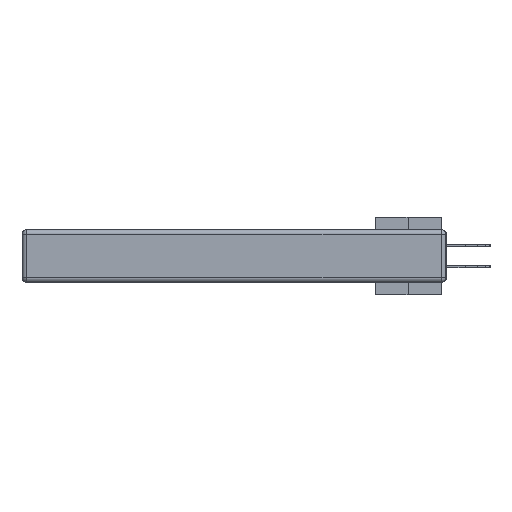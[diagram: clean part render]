
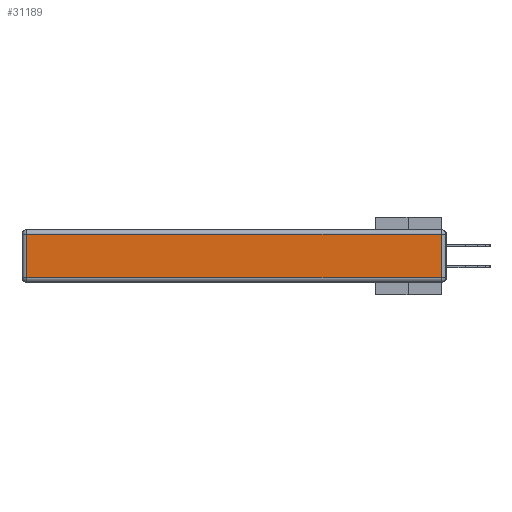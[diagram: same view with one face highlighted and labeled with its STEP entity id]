
A CAD part, left-side view. The second image highlights one B-rep face of the part: STEP entity #31189.
In plain terms, the highlighted planar face has unit normal (-1, 0, 0).
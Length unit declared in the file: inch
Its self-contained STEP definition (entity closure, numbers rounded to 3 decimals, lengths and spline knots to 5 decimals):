
#1089 = CARTESIAN_POINT ( 'NONE',  ( 0., 0.03, -0.03 ) ) ;
#5741 = EDGE_CURVE ( 'NONE', #34236, #11768, #42844, .T. ) ;
#6811 = AXIS2_PLACEMENT_3D ( 'NONE', #33248, #10480, #29893 ) ;
#7391 = EDGE_CURVE ( 'NONE', #47615, #34236, #17768, .T. ) ;
#8112 = CARTESIAN_POINT ( 'NONE',  ( 0., 2.72, -0.313 ) ) ;
#8510 = DIRECTION ( 'NONE',  ( 0., 0., -1. ) ) ;
#8894 = VECTOR ( 'NONE', #30757, 39.37008 ) ;
#10480 = DIRECTION ( 'NONE',  ( -1., 0., 0. ) ) ;
#10855 = DIRECTION ( 'NONE',  ( 0., 1., 0. ) ) ;
#11768 = VERTEX_POINT ( 'NONE', #32466 ) ;
#12795 = LINE ( 'NONE', #27780, #28231 ) ;
#14341 = CARTESIAN_POINT ( 'NONE',  ( 0., 2.75, -0.03 ) ) ;
#14441 = PLANE ( 'NONE',  #6811 ) ;
#15996 = VECTOR ( 'NONE', #45550, 39.37008 ) ;
#16296 = EDGE_LOOP ( 'NONE', ( #17595, #16425, #37503, #38495 ) ) ;
#16425 = ORIENTED_EDGE ( 'NONE', *, *, #7391, .T. ) ;
#17595 = ORIENTED_EDGE ( 'NONE', *, *, #44798, .T. ) ;
#17768 = LINE ( 'NONE', #42056, #8894 ) ;
#23877 = EDGE_CURVE ( 'NONE', #11768, #44087, #12795, .T. ) ;
#25041 = VECTOR ( 'NONE', #10855, 39.37008 ) ;
#27780 = CARTESIAN_POINT ( 'NONE',  ( 0., 2.72, -0.343 ) ) ;
#28231 = VECTOR ( 'NONE', #8510, 39.37008 ) ;
#28425 = FACE_OUTER_BOUND ( 'NONE', #16296, .T. ) ;
#29893 = DIRECTION ( 'NONE',  ( 0., 0., 1. ) ) ;
#30757 = DIRECTION ( 'NONE',  ( 0., 0., 1. ) ) ;
#31189 = ADVANCED_FACE ( 'NONE', ( #28425 ), #14441, .T. ) ;
#32466 = CARTESIAN_POINT ( 'NONE',  ( 0., 2.72, -0.03 ) ) ;
#33248 = CARTESIAN_POINT ( 'NONE',  ( 0., 0., -0.343 ) ) ;
#34236 = VERTEX_POINT ( 'NONE', #1089 ) ;
#37503 = ORIENTED_EDGE ( 'NONE', *, *, #5741, .T. ) ;
#37686 = CARTESIAN_POINT ( 'NONE',  ( 0., 0.03, -0.313 ) ) ;
#37990 = LINE ( 'NONE', #42088, #15996 ) ;
#38495 = ORIENTED_EDGE ( 'NONE', *, *, #23877, .T. ) ;
#42056 = CARTESIAN_POINT ( 'NONE',  ( 0., 0.03, -0.343 ) ) ;
#42088 = CARTESIAN_POINT ( 'NONE',  ( 0., 0., -0.313 ) ) ;
#42844 = LINE ( 'NONE', #14341, #25041 ) ;
#44087 = VERTEX_POINT ( 'NONE', #8112 ) ;
#44798 = EDGE_CURVE ( 'NONE', #44087, #47615, #37990, .T. ) ;
#45550 = DIRECTION ( 'NONE',  ( 0., -1., 0. ) ) ;
#47615 = VERTEX_POINT ( 'NONE', #37686 ) ;
